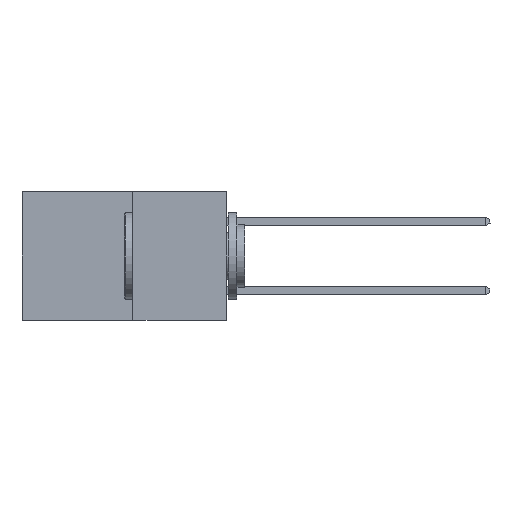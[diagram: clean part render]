
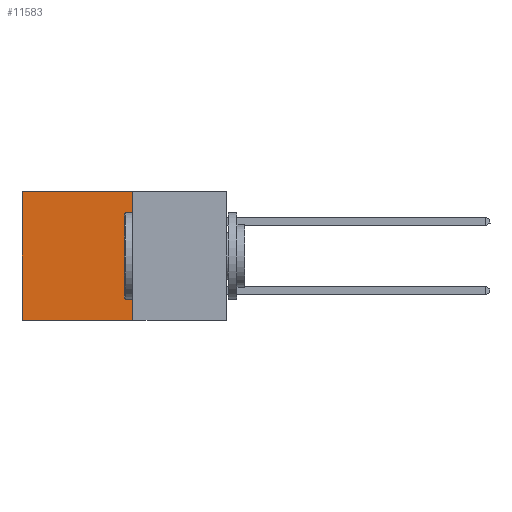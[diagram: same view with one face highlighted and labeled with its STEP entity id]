
A CAD part, left-side view. The second image highlights one B-rep face of the part: STEP entity #11583.
In plain terms, the highlighted planar face has unit normal (-1, 0, 0).
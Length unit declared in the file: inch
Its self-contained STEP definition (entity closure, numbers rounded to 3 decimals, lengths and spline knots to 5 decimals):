
#31 = DIRECTION ( 'NONE',  ( 0., 0., -1. ) ) ;
#215 = VECTOR ( 'NONE', #4641, 39.37008 ) ;
#1618 = CARTESIAN_POINT ( 'NONE',  ( 0.277, 0.59, -0.37 ) ) ;
#1891 = EDGE_LOOP ( 'NONE', ( #4855, #7398, #10183, #10479 ) ) ;
#2086 = LINE ( 'NONE', #10362, #11247 ) ;
#2534 = DIRECTION ( 'NONE',  ( 0., 0., -1. ) ) ;
#2666 = LINE ( 'NONE', #8359, #7436 ) ;
#4641 = DIRECTION ( 'NONE',  ( 0., 1., 0. ) ) ;
#4671 = AXIS2_PLACEMENT_3D ( 'NONE', #11280, #5616, #31 ) ;
#4855 = ORIENTED_EDGE ( 'NONE', *, *, #12063, .T. ) ;
#5051 = VERTEX_POINT ( 'NONE', #7862 ) ;
#5616 = DIRECTION ( 'NONE',  ( 1., 0., 0. ) ) ;
#6188 = CARTESIAN_POINT ( 'NONE',  ( 0.277, 0.27, 0. ) ) ;
#6768 = VECTOR ( 'NONE', #2534, 39.37008 ) ;
#7398 = ORIENTED_EDGE ( 'NONE', *, *, #10335, .F. ) ;
#7436 = VECTOR ( 'NONE', #9292, 39.37008 ) ;
#7649 = EDGE_CURVE ( 'NONE', #10034, #11038, #7732, .T. ) ;
#7732 = LINE ( 'NONE', #11252, #215 ) ;
#7774 = CARTESIAN_POINT ( 'NONE',  ( 0.277, 0.59, 0. ) ) ;
#7862 = CARTESIAN_POINT ( 'NONE',  ( 0.277, 0.59, -0.37 ) ) ;
#8081 = CARTESIAN_POINT ( 'NONE',  ( 0.277, 0.27, -0.37 ) ) ;
#8359 = CARTESIAN_POINT ( 'NONE',  ( 0.277, 0.27, -0.37 ) ) ;
#8495 = PLANE ( 'NONE',  #4671 ) ;
#9292 = DIRECTION ( 'NONE',  ( 0., 0., -1. ) ) ;
#9545 = EDGE_CURVE ( 'NONE', #10034, #10564, #2666, .T. ) ;
#9600 = LINE ( 'NONE', #1618, #6768 ) ;
#9886 = FACE_OUTER_BOUND ( 'NONE', #1891, .T. ) ;
#10034 = VERTEX_POINT ( 'NONE', #6188 ) ;
#10183 = ORIENTED_EDGE ( 'NONE', *, *, #9545, .F. ) ;
#10335 = EDGE_CURVE ( 'NONE', #10564, #5051, #2086, .T. ) ;
#10362 = CARTESIAN_POINT ( 'NONE',  ( 0.277, 0.27, -0.37 ) ) ;
#10479 = ORIENTED_EDGE ( 'NONE', *, *, #7649, .T. ) ;
#10564 = VERTEX_POINT ( 'NONE', #8081 ) ;
#11038 = VERTEX_POINT ( 'NONE', #7774 ) ;
#11247 = VECTOR ( 'NONE', #11305, 39.37008 ) ;
#11252 = CARTESIAN_POINT ( 'NONE',  ( 0.277, 0.27, 0. ) ) ;
#11280 = CARTESIAN_POINT ( 'NONE',  ( 0.277, 0.27, -0.37 ) ) ;
#11305 = DIRECTION ( 'NONE',  ( 0., 1., 0. ) ) ;
#11583 = ADVANCED_FACE ( 'NONE', ( #9886 ), #8495, .F. ) ;
#12063 = EDGE_CURVE ( 'NONE', #11038, #5051, #9600, .T. ) ;
